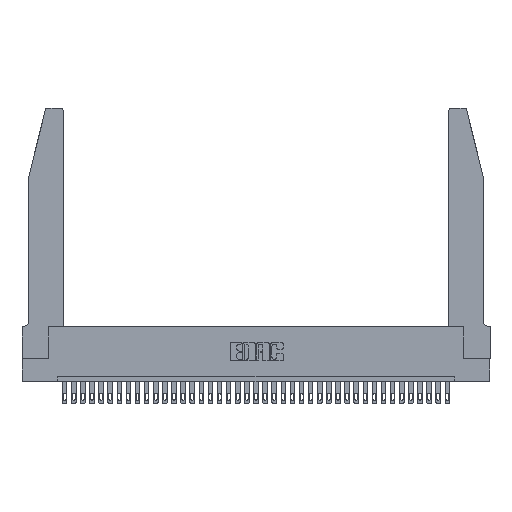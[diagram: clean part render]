
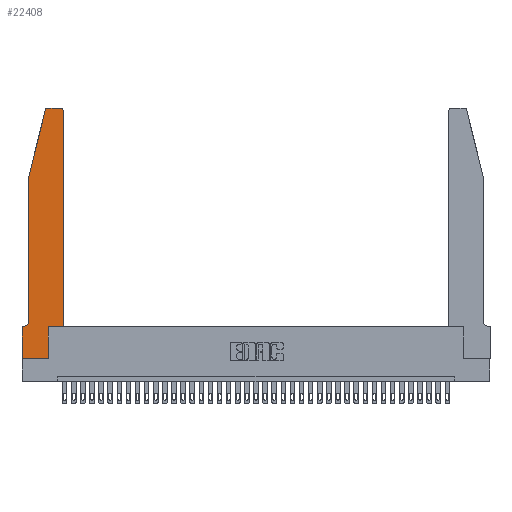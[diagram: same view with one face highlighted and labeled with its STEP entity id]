
A CAD part, top view. The second image highlights one B-rep face of the part: STEP entity #22408.
In plain terms, the highlighted planar face has unit normal (0, 0, 1).
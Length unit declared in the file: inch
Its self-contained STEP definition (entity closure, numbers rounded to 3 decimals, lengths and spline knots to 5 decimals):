
#501 = DIRECTION ( 'NONE',  ( -0.239, -0.971, 0. ) ) ;
#682 = ORIENTED_EDGE ( 'NONE', *, *, #17835, .T. ) ;
#1191 = DIRECTION ( 'NONE',  ( -1., 0., 0. ) ) ;
#1361 = VERTEX_POINT ( 'NONE', #10212 ) ;
#1490 = VECTOR ( 'NONE', #29789, 39.37008 ) ;
#2408 = DIRECTION ( 'NONE',  ( 0., 0., 1. ) ) ;
#2572 = LINE ( 'NONE', #23716, #18606 ) ;
#3458 = CARTESIAN_POINT ( 'NONE',  ( 0.4505, 2.72, 0.37 ) ) ;
#3770 = DIRECTION ( 'NONE',  ( 0., 1., 0. ) ) ;
#4227 = EDGE_CURVE ( 'NONE', #7557, #20200, #35784, .T. ) ;
#4516 = EDGE_CURVE ( 'NONE', #1361, #11251, #9040, .T. ) ;
#4891 = VERTEX_POINT ( 'NONE', #23282 ) ;
#5391 = CIRCLE ( 'NONE', #20550, 0.03 ) ;
#5861 = LINE ( 'NONE', #23460, #25471 ) ;
#6105 = EDGE_LOOP ( 'NONE', ( #35938, #27308, #682, #36357, #25410, #26517, #11857, #31408, #15980, #35858, #13601, #18949 ) ) ;
#6245 = EDGE_CURVE ( 'NONE', #17142, #23361, #5391, .T. ) ;
#6250 = CARTESIAN_POINT ( 'NONE',  ( 0.0755, 0.35, 0.37 ) ) ;
#7557 = VERTEX_POINT ( 'NONE', #26640 ) ;
#8969 = DIRECTION ( 'NONE',  ( 1., 0., 0. ) ) ;
#9040 = LINE ( 'NONE', #24422, #1490 ) ;
#10212 = CARTESIAN_POINT ( 'NONE',  ( 0.0755, 2., 0.37 ) ) ;
#10906 = EDGE_CURVE ( 'NONE', #4891, #20728, #18807, .T. ) ;
#11251 = VERTEX_POINT ( 'NONE', #19659 ) ;
#11511 = EDGE_CURVE ( 'NONE', #24172, #35528, #14251, .T. ) ;
#11682 = CARTESIAN_POINT ( 'NONE',  ( 0.2865, 0.35, 0.37 ) ) ;
#11857 = ORIENTED_EDGE ( 'NONE', *, *, #11511, .T. ) ;
#13601 = ORIENTED_EDGE ( 'NONE', *, *, #4227, .T. ) ;
#13747 = CIRCLE ( 'NONE', #34723, 0.03 ) ;
#14251 = LINE ( 'NONE', #18984, #18284 ) ;
#14741 = FACE_OUTER_BOUND ( 'NONE', #6105, .T. ) ;
#14958 = CIRCLE ( 'NONE', #25110, 0.07 ) ;
#15820 = DIRECTION ( 'NONE',  ( -1., 0., 0. ) ) ;
#15961 = VECTOR ( 'NONE', #15820, 39.37008 ) ;
#15980 = ORIENTED_EDGE ( 'NONE', *, *, #10906, .T. ) ;
#16436 = LINE ( 'NONE', #6250, #15961 ) ;
#16473 = CARTESIAN_POINT ( 'NONE',  ( 0.4205, 2.75, 0.37 ) ) ;
#16525 = CARTESIAN_POINT ( 'NONE',  ( 0.0055, 0.42, 0.37 ) ) ;
#16762 = DIRECTION ( 'NONE',  ( -1., 0., 0. ) ) ;
#17142 = VERTEX_POINT ( 'NONE', #25723 ) ;
#17209 = EDGE_CURVE ( 'NONE', #20728, #7557, #5861, .T. ) ;
#17687 = DIRECTION ( 'NONE',  ( 0., 0., 1. ) ) ;
#17835 = EDGE_CURVE ( 'NONE', #23361, #1361, #34344, .T. ) ;
#18284 = VECTOR ( 'NONE', #25053, 39.37008 ) ;
#18606 = VECTOR ( 'NONE', #1191, 39.37008 ) ;
#18807 = LINE ( 'NONE', #11682, #32607 ) ;
#18949 = ORIENTED_EDGE ( 'NONE', *, *, #36748, .T. ) ;
#18984 = CARTESIAN_POINT ( 'NONE',  ( 0., 0., 0.37 ) ) ;
#19337 = PLANE ( 'NONE',  #28490 ) ;
#19455 = CARTESIAN_POINT ( 'NONE',  ( 0., 0., 0.37 ) ) ;
#19539 = EDGE_CURVE ( 'NONE', #35162, #24172, #16436, .T. ) ;
#19659 = CARTESIAN_POINT ( 'NONE',  ( 0.0755, 0.42, 0.37 ) ) ;
#20200 = VERTEX_POINT ( 'NONE', #3458 ) ;
#20295 = EDGE_CURVE ( 'NONE', #24313, #17142, #2572, .T. ) ;
#20388 = EDGE_CURVE ( 'NONE', #11251, #35162, #14958, .T. ) ;
#20511 = VECTOR ( 'NONE', #27676, 39.37008 ) ;
#20550 = AXIS2_PLACEMENT_3D ( 'NONE', #23124, #17687, #8969 ) ;
#20728 = VERTEX_POINT ( 'NONE', #35256 ) ;
#21936 = VECTOR ( 'NONE', #24578, 39.37008 ) ;
#22213 = DIRECTION ( 'NONE',  ( 1., 0., 0. ) ) ;
#22408 = ADVANCED_FACE ( 'NONE', ( #14741 ), #19337, .T. ) ;
#23124 = CARTESIAN_POINT ( 'NONE',  ( 0.284, 2.72, 0.37 ) ) ;
#23282 = CARTESIAN_POINT ( 'NONE',  ( 0.2865, 0., 0.37 ) ) ;
#23343 = DIRECTION ( 'NONE',  ( 1., 0., 0. ) ) ;
#23361 = VERTEX_POINT ( 'NONE', #33432 ) ;
#23460 = CARTESIAN_POINT ( 'NONE',  ( 0.4505, 0.35, 0.37 ) ) ;
#23716 = CARTESIAN_POINT ( 'NONE',  ( 0.2605, 2.75, 0.37 ) ) ;
#24172 = VERTEX_POINT ( 'NONE', #26544 ) ;
#24313 = VERTEX_POINT ( 'NONE', #16473 ) ;
#24422 = CARTESIAN_POINT ( 'NONE',  ( 0.0755, 2., 0.37 ) ) ;
#24515 = VECTOR ( 'NONE', #501, 39.37008 ) ;
#24578 = DIRECTION ( 'NONE',  ( 0., 1., 0. ) ) ;
#25053 = DIRECTION ( 'NONE',  ( 0., -1., 0. ) ) ;
#25110 = AXIS2_PLACEMENT_3D ( 'NONE', #16525, #36457, #16762 ) ;
#25410 = ORIENTED_EDGE ( 'NONE', *, *, #20388, .T. ) ;
#25471 = VECTOR ( 'NONE', #23343, 39.37008 ) ;
#25723 = CARTESIAN_POINT ( 'NONE',  ( 0.284, 2.75, 0.37 ) ) ;
#26517 = ORIENTED_EDGE ( 'NONE', *, *, #19539, .T. ) ;
#26544 = CARTESIAN_POINT ( 'NONE',  ( 0., 0.35, 0.37 ) ) ;
#26640 = CARTESIAN_POINT ( 'NONE',  ( 0.4505, 0.35, 0.37 ) ) ;
#27308 = ORIENTED_EDGE ( 'NONE', *, *, #6245, .T. ) ;
#27565 = CARTESIAN_POINT ( 'NONE',  ( 0.4505, 0.35, 0.37 ) ) ;
#27676 = DIRECTION ( 'NONE',  ( 1., 0., 0. ) ) ;
#28490 = AXIS2_PLACEMENT_3D ( 'NONE', #33666, #2408, #33782 ) ;
#29656 = CARTESIAN_POINT ( 'NONE',  ( 0.0055, 0.35, 0.37 ) ) ;
#29789 = DIRECTION ( 'NONE',  ( 0., -1., 0. ) ) ;
#31186 = CARTESIAN_POINT ( 'NONE',  ( 0.4205, 2.72, 0.37 ) ) ;
#31408 = ORIENTED_EDGE ( 'NONE', *, *, #35432, .T. ) ;
#32607 = VECTOR ( 'NONE', #3770, 39.37008 ) ;
#33432 = CARTESIAN_POINT ( 'NONE',  ( 0.25487, 2.72718, 0.37 ) ) ;
#33578 = DIRECTION ( 'NONE',  ( 0., 0., 1. ) ) ;
#33666 = CARTESIAN_POINT ( 'NONE',  ( 0., 0.35, 0.37 ) ) ;
#33782 = DIRECTION ( 'NONE',  ( 1., 0., 0. ) ) ;
#34344 = LINE ( 'NONE', #34774, #24515 ) ;
#34370 = LINE ( 'NONE', #19455, #20511 ) ;
#34723 = AXIS2_PLACEMENT_3D ( 'NONE', #31186, #33578, #22213 ) ;
#34774 = CARTESIAN_POINT ( 'NONE',  ( 0.0755, 2., 0.37 ) ) ;
#35162 = VERTEX_POINT ( 'NONE', #29656 ) ;
#35256 = CARTESIAN_POINT ( 'NONE',  ( 0.2865, 0.35, 0.37 ) ) ;
#35432 = EDGE_CURVE ( 'NONE', #35528, #4891, #34370, .T. ) ;
#35528 = VERTEX_POINT ( 'NONE', #36158 ) ;
#35784 = LINE ( 'NONE', #27565, #21936 ) ;
#35858 = ORIENTED_EDGE ( 'NONE', *, *, #17209, .T. ) ;
#35938 = ORIENTED_EDGE ( 'NONE', *, *, #20295, .T. ) ;
#36158 = CARTESIAN_POINT ( 'NONE',  ( 0., 0., 0.37 ) ) ;
#36357 = ORIENTED_EDGE ( 'NONE', *, *, #4516, .T. ) ;
#36457 = DIRECTION ( 'NONE',  ( 0., 0., -1. ) ) ;
#36748 = EDGE_CURVE ( 'NONE', #20200, #24313, #13747, .T. ) ;
